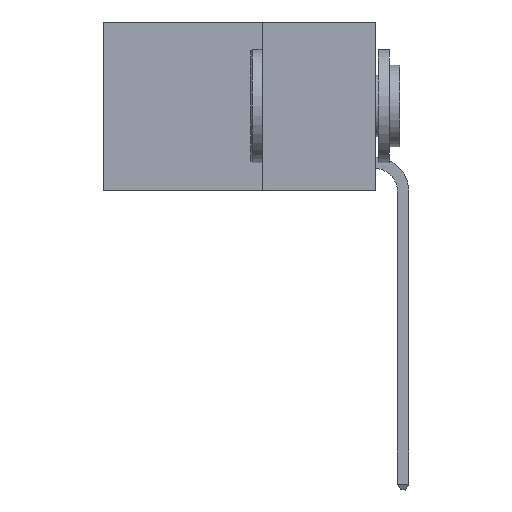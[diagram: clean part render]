
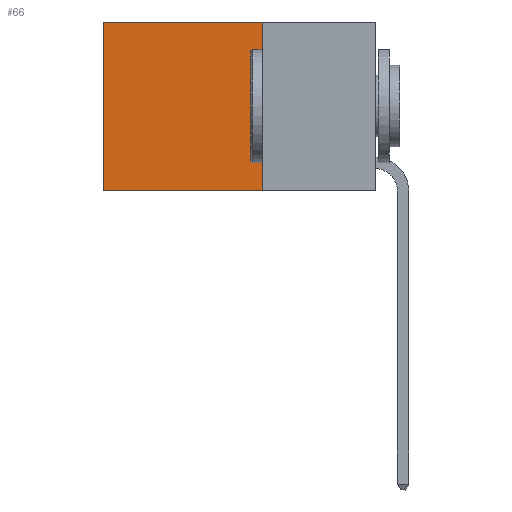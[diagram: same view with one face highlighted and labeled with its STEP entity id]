
A CAD part, left-side view. The second image highlights one B-rep face of the part: STEP entity #66.
In plain terms, the highlighted planar face has unit normal (-1, 0, 0).
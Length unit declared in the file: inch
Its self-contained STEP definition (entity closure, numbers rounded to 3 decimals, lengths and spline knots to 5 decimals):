
#66 = ADVANCED_FACE ( 'NONE', ( #7092 ), #6377, .F. ) ;
#345 = VERTEX_POINT ( 'NONE', #8065 ) ;
#679 = VECTOR ( 'NONE', #8895, 39.37008 ) ;
#871 = LINE ( 'NONE', #4075, #4929 ) ;
#1041 = CARTESIAN_POINT ( 'NONE',  ( 0.2625, 0.25, -0.37 ) ) ;
#1508 = VECTOR ( 'NONE', #1884, 39.37008 ) ;
#1845 = VERTEX_POINT ( 'NONE', #9781 ) ;
#1884 = DIRECTION ( 'NONE',  ( 0., 1., 0. ) ) ;
#2189 = ORIENTED_EDGE ( 'NONE', *, *, #9687, .T. ) ;
#2793 = CARTESIAN_POINT ( 'NONE',  ( 0.2625, 0.6, 0. ) ) ;
#2993 = CARTESIAN_POINT ( 'NONE',  ( 0.2625, 0.25, 0. ) ) ;
#3814 = AXIS2_PLACEMENT_3D ( 'NONE', #5884, #6847, #9185 ) ;
#3832 = VERTEX_POINT ( 'NONE', #2793 ) ;
#4075 = CARTESIAN_POINT ( 'NONE',  ( 0.2625, 0.25, 0. ) ) ;
#4089 = ORIENTED_EDGE ( 'NONE', *, *, #5875, .F. ) ;
#4436 = EDGE_CURVE ( 'NONE', #1845, #345, #7686, .T. ) ;
#4497 = DIRECTION ( 'NONE',  ( 0., 0., -1. ) ) ;
#4929 = VECTOR ( 'NONE', #6344, 39.37008 ) ;
#4985 = VECTOR ( 'NONE', #4497, 39.37008 ) ;
#5216 = LINE ( 'NONE', #2993, #679 ) ;
#5358 = VERTEX_POINT ( 'NONE', #6288 ) ;
#5875 = EDGE_CURVE ( 'NONE', #5358, #1845, #5216, .T. ) ;
#5884 = CARTESIAN_POINT ( 'NONE',  ( 0.2625, 0.25, 0. ) ) ;
#6288 = CARTESIAN_POINT ( 'NONE',  ( 0.2625, 0.25, 0. ) ) ;
#6321 = EDGE_CURVE ( 'NONE', #3832, #345, #7228, .T. ) ;
#6344 = DIRECTION ( 'NONE',  ( 0., 1., 0. ) ) ;
#6377 = PLANE ( 'NONE',  #3814 ) ;
#6537 = ORIENTED_EDGE ( 'NONE', *, *, #4436, .F. ) ;
#6801 = ORIENTED_EDGE ( 'NONE', *, *, #6321, .T. ) ;
#6847 = DIRECTION ( 'NONE',  ( 1., 0., 0. ) ) ;
#7092 = FACE_OUTER_BOUND ( 'NONE', #8303, .T. ) ;
#7228 = LINE ( 'NONE', #8800, #4985 ) ;
#7686 = LINE ( 'NONE', #1041, #1508 ) ;
#8065 = CARTESIAN_POINT ( 'NONE',  ( 0.2625, 0.6, -0.37 ) ) ;
#8303 = EDGE_LOOP ( 'NONE', ( #6801, #6537, #4089, #2189 ) ) ;
#8800 = CARTESIAN_POINT ( 'NONE',  ( 0.2625, 0.6, 0. ) ) ;
#8895 = DIRECTION ( 'NONE',  ( 0., 0., -1. ) ) ;
#9185 = DIRECTION ( 'NONE',  ( 0., 0., -1. ) ) ;
#9687 = EDGE_CURVE ( 'NONE', #5358, #3832, #871, .T. ) ;
#9781 = CARTESIAN_POINT ( 'NONE',  ( 0.2625, 0.25, -0.37 ) ) ;
